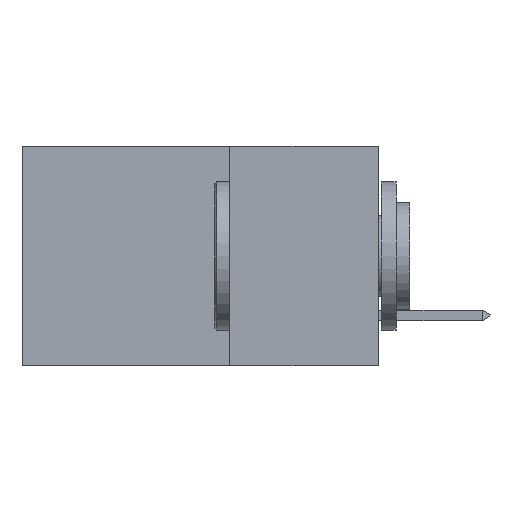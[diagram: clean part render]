
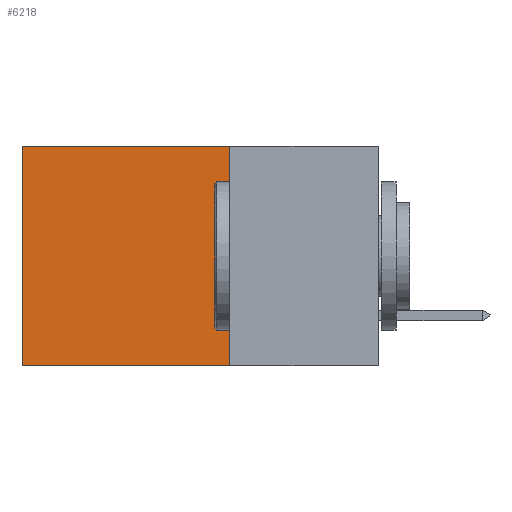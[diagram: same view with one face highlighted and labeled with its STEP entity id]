
A CAD part, left-side view. The second image highlights one B-rep face of the part: STEP entity #6218.
In plain terms, the highlighted planar face has unit normal (-1, 0, 0).
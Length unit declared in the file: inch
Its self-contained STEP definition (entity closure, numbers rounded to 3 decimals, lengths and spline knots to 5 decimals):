
#17 = LINE ( 'NONE', #17936, #9150 ) ;
#31 = LINE ( 'NONE', #19636, #23060 ) ;
#1549 = VECTOR ( 'NONE', #12963, 39.37008 ) ;
#2532 = PLANE ( 'NONE',  #25041 ) ;
#4038 = EDGE_CURVE ( 'NONE', #13541, #5611, #17, .T. ) ;
#4598 = CARTESIAN_POINT ( 'NONE',  ( 0.2615, 0.25, -0.37 ) ) ;
#5274 = LINE ( 'NONE', #7477, #6435 ) ;
#5506 = EDGE_CURVE ( 'NONE', #22470, #9598, #5274, .T. ) ;
#5611 = VERTEX_POINT ( 'NONE', #25293 ) ;
#6218 = ADVANCED_FACE ( 'NONE', ( #18151 ), #2532, .F. ) ;
#6259 = CARTESIAN_POINT ( 'NONE',  ( 0.2615, 0.6, 0. ) ) ;
#6435 = VECTOR ( 'NONE', #25420, 39.37008 ) ;
#6825 = CARTESIAN_POINT ( 'NONE',  ( 0.2615, 0.6, -0.37 ) ) ;
#6858 = EDGE_LOOP ( 'NONE', ( #14801, #10420, #20895, #21213 ) ) ;
#7477 = CARTESIAN_POINT ( 'NONE',  ( 0.2615, 0.6, -0.37 ) ) ;
#8740 = DIRECTION ( 'NONE',  ( 0., 0., -1. ) ) ;
#9150 = VECTOR ( 'NONE', #16119, 39.37008 ) ;
#9598 = VERTEX_POINT ( 'NONE', #6825 ) ;
#10420 = ORIENTED_EDGE ( 'NONE', *, *, #10687, .F. ) ;
#10687 = EDGE_CURVE ( 'NONE', #5611, #9598, #18639, .T. ) ;
#11236 = DIRECTION ( 'NONE',  ( 0., 1., 0. ) ) ;
#12577 = CARTESIAN_POINT ( 'NONE',  ( 0.2615, 0.25, -0.37 ) ) ;
#12963 = DIRECTION ( 'NONE',  ( 0., 1., 0. ) ) ;
#13541 = VERTEX_POINT ( 'NONE', #23636 ) ;
#14801 = ORIENTED_EDGE ( 'NONE', *, *, #5506, .T. ) ;
#16119 = DIRECTION ( 'NONE',  ( 0., 0., -1. ) ) ;
#17936 = CARTESIAN_POINT ( 'NONE',  ( 0.2615, 0.25, -0.37 ) ) ;
#18151 = FACE_OUTER_BOUND ( 'NONE', #6858, .T. ) ;
#18639 = LINE ( 'NONE', #12577, #1549 ) ;
#19636 = CARTESIAN_POINT ( 'NONE',  ( 0.2615, 0.25, 0. ) ) ;
#20485 = DIRECTION ( 'NONE',  ( 1., 0., 0. ) ) ;
#20895 = ORIENTED_EDGE ( 'NONE', *, *, #4038, .F. ) ;
#21213 = ORIENTED_EDGE ( 'NONE', *, *, #25185, .T. ) ;
#22470 = VERTEX_POINT ( 'NONE', #6259 ) ;
#23060 = VECTOR ( 'NONE', #11236, 39.37008 ) ;
#23636 = CARTESIAN_POINT ( 'NONE',  ( 0.2615, 0.25, 0. ) ) ;
#25041 = AXIS2_PLACEMENT_3D ( 'NONE', #4598, #20485, #8740 ) ;
#25185 = EDGE_CURVE ( 'NONE', #13541, #22470, #31, .T. ) ;
#25293 = CARTESIAN_POINT ( 'NONE',  ( 0.2615, 0.25, -0.37 ) ) ;
#25420 = DIRECTION ( 'NONE',  ( 0., 0., -1. ) ) ;
